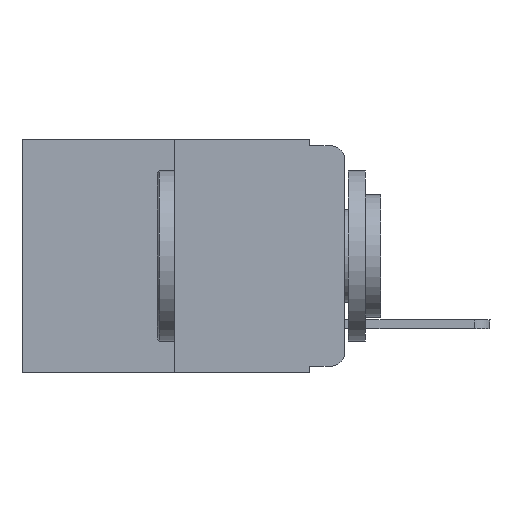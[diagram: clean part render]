
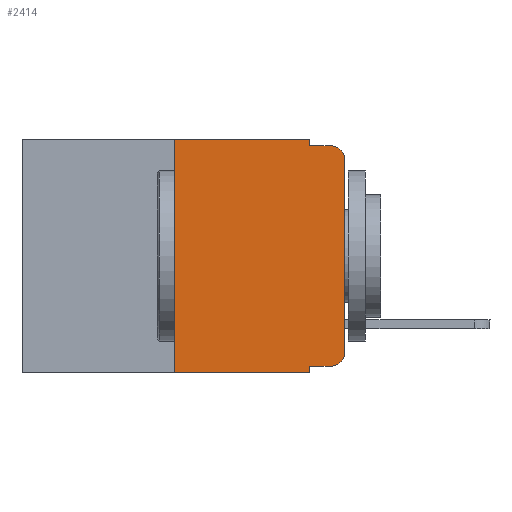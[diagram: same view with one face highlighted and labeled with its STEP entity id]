
A CAD part, left-side view. The second image highlights one B-rep face of the part: STEP entity #2414.
In plain terms, the highlighted planar face has unit normal (-1, 0, 0).
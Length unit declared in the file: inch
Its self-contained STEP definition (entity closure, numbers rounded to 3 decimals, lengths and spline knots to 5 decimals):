
#46 = LINE ( 'NONE', #21617, #14237 ) ;
#637 = EDGE_CURVE ( 'NONE', #17600, #7839, #819, .T. ) ;
#819 = LINE ( 'NONE', #11331, #10467 ) ;
#971 = CARTESIAN_POINT ( 'NONE',  ( 0., 0.051, 0. ) ) ;
#1247 = DIRECTION ( 'NONE',  ( 0., -1., 0. ) ) ;
#1508 = LINE ( 'NONE', #14892, #14512 ) ;
#1557 = CARTESIAN_POINT ( 'NONE',  ( 0., 0., -0.313 ) ) ;
#1723 = ORIENTED_EDGE ( 'NONE', *, *, #7116, .F. ) ;
#2285 = VECTOR ( 'NONE', #19127, 39.37008 ) ;
#2287 = CARTESIAN_POINT ( 'NONE',  ( 0., 0.02, -0.03 ) ) ;
#2414 = ADVANCED_FACE ( 'NONE', ( #19312 ), #16241, .F. ) ;
#2443 = CARTESIAN_POINT ( 'NONE',  ( 0., 0.051, 0. ) ) ;
#3305 = VECTOR ( 'NONE', #5601, 39.37008 ) ;
#3357 = CARTESIAN_POINT ( 'NONE',  ( 0., 0.051, -0.343 ) ) ;
#3943 = EDGE_CURVE ( 'NONE', #17600, #12637, #16001, .T. ) ;
#4722 = CARTESIAN_POINT ( 'NONE',  ( 0., 0.051, -0.01 ) ) ;
#4824 = VERTEX_POINT ( 'NONE', #1557 ) ;
#4879 = VERTEX_POINT ( 'NONE', #4722 ) ;
#4895 = CARTESIAN_POINT ( 'NONE',  ( 0., 0.25, -0.343 ) ) ;
#5036 = VERTEX_POINT ( 'NONE', #17014 ) ;
#5347 = EDGE_LOOP ( 'NONE', ( #19620, #7725, #9816, #8120, #1723, #7986, #13422, #17376, #12978, #16929 ) ) ;
#5351 = EDGE_CURVE ( 'NONE', #7839, #4824, #8330, .T. ) ;
#5516 = AXIS2_PLACEMENT_3D ( 'NONE', #12047, #6700, #10538 ) ;
#5601 = DIRECTION ( 'NONE',  ( 0., 0., -1. ) ) ;
#5611 = EDGE_CURVE ( 'NONE', #13823, #4879, #17302, .T. ) ;
#6069 = DIRECTION ( 'NONE',  ( 0., 0., -1. ) ) ;
#6652 = DIRECTION ( 'NONE',  ( 0., 0., 1. ) ) ;
#6700 = DIRECTION ( 'NONE',  ( -1., 0., 0. ) ) ;
#6848 = VECTOR ( 'NONE', #20516, 39.37008 ) ;
#7116 = EDGE_CURVE ( 'NONE', #13870, #13823, #14210, .T. ) ;
#7242 = CARTESIAN_POINT ( 'NONE',  ( 0., 0.051, 0. ) ) ;
#7564 = DIRECTION ( 'NONE',  ( -1., 0., 0. ) ) ;
#7698 = CARTESIAN_POINT ( 'NONE',  ( 0., 0.25, 0. ) ) ;
#7725 = ORIENTED_EDGE ( 'NONE', *, *, #16292, .T. ) ;
#7839 = VERTEX_POINT ( 'NONE', #17001 ) ;
#7986 = ORIENTED_EDGE ( 'NONE', *, *, #19945, .F. ) ;
#8120 = ORIENTED_EDGE ( 'NONE', *, *, #5611, .F. ) ;
#8330 = CIRCLE ( 'NONE', #5516, 0.02 ) ;
#9600 = VECTOR ( 'NONE', #17447, 39.37008 ) ;
#9816 = ORIENTED_EDGE ( 'NONE', *, *, #15252, .F. ) ;
#9851 = AXIS2_PLACEMENT_3D ( 'NONE', #16040, #21043, #6069 ) ;
#9852 = VERTEX_POINT ( 'NONE', #4895 ) ;
#10467 = VECTOR ( 'NONE', #1247, 39.37008 ) ;
#10491 = CARTESIAN_POINT ( 'NONE',  ( 0., 0.473, -0.343 ) ) ;
#10538 = DIRECTION ( 'NONE',  ( 0., 0., -1. ) ) ;
#10631 = DIRECTION ( 'NONE',  ( 0., 0., -1. ) ) ;
#10908 = LINE ( 'NONE', #10491, #6848 ) ;
#11331 = CARTESIAN_POINT ( 'NONE',  ( 0., 0.051, -0.333 ) ) ;
#11449 = EDGE_CURVE ( 'NONE', #9852, #12637, #10908, .T. ) ;
#11863 = CARTESIAN_POINT ( 'NONE',  ( 0., 0.051, -0.333 ) ) ;
#12047 = CARTESIAN_POINT ( 'NONE',  ( 0., 0.02, -0.313 ) ) ;
#12450 = CARTESIAN_POINT ( 'NONE',  ( 0., 0.473, 0. ) ) ;
#12637 = VERTEX_POINT ( 'NONE', #3357 ) ;
#12693 = EDGE_CURVE ( 'NONE', #4824, #5036, #46, .T. ) ;
#12978 = ORIENTED_EDGE ( 'NONE', *, *, #637, .T. ) ;
#13084 = CARTESIAN_POINT ( 'NONE',  ( 0., 0.02, -0.01 ) ) ;
#13422 = ORIENTED_EDGE ( 'NONE', *, *, #11449, .T. ) ;
#13491 = AXIS2_PLACEMENT_3D ( 'NONE', #2287, #7564, #10631 ) ;
#13823 = VERTEX_POINT ( 'NONE', #971 ) ;
#13837 = LINE ( 'NONE', #14154, #17056 ) ;
#13870 = VERTEX_POINT ( 'NONE', #7698 ) ;
#13951 = DIRECTION ( 'NONE',  ( 0., 0., 1. ) ) ;
#14154 = CARTESIAN_POINT ( 'NONE',  ( 0., 0.25, 0. ) ) ;
#14210 = LINE ( 'NONE', #12450, #2285 ) ;
#14237 = VECTOR ( 'NONE', #6652, 39.37008 ) ;
#14512 = VECTOR ( 'NONE', #15214, 39.37008 ) ;
#14892 = CARTESIAN_POINT ( 'NONE',  ( 0., 0.051, -0.01 ) ) ;
#15214 = DIRECTION ( 'NONE',  ( 0., -1., 0. ) ) ;
#15252 = EDGE_CURVE ( 'NONE', #4879, #16889, #1508, .T. ) ;
#16001 = LINE ( 'NONE', #2443, #9600 ) ;
#16040 = CARTESIAN_POINT ( 'NONE',  ( 0., 0.473, 0. ) ) ;
#16241 = PLANE ( 'NONE',  #9851 ) ;
#16292 = EDGE_CURVE ( 'NONE', #5036, #16889, #21164, .T. ) ;
#16889 = VERTEX_POINT ( 'NONE', #13084 ) ;
#16929 = ORIENTED_EDGE ( 'NONE', *, *, #5351, .T. ) ;
#17001 = CARTESIAN_POINT ( 'NONE',  ( 0., 0.02, -0.333 ) ) ;
#17014 = CARTESIAN_POINT ( 'NONE',  ( 0., 0., -0.03 ) ) ;
#17056 = VECTOR ( 'NONE', #13951, 39.37008 ) ;
#17302 = LINE ( 'NONE', #7242, #3305 ) ;
#17376 = ORIENTED_EDGE ( 'NONE', *, *, #3943, .F. ) ;
#17447 = DIRECTION ( 'NONE',  ( 0., 0., -1. ) ) ;
#17600 = VERTEX_POINT ( 'NONE', #11863 ) ;
#19127 = DIRECTION ( 'NONE',  ( 0., -1., 0. ) ) ;
#19312 = FACE_OUTER_BOUND ( 'NONE', #5347, .T. ) ;
#19620 = ORIENTED_EDGE ( 'NONE', *, *, #12693, .T. ) ;
#19945 = EDGE_CURVE ( 'NONE', #9852, #13870, #13837, .T. ) ;
#20516 = DIRECTION ( 'NONE',  ( 0., -1., 0. ) ) ;
#21043 = DIRECTION ( 'NONE',  ( 1., 0., 0. ) ) ;
#21164 = CIRCLE ( 'NONE', #13491, 0.02 ) ;
#21617 = CARTESIAN_POINT ( 'NONE',  ( 0., 0., 0. ) ) ;
